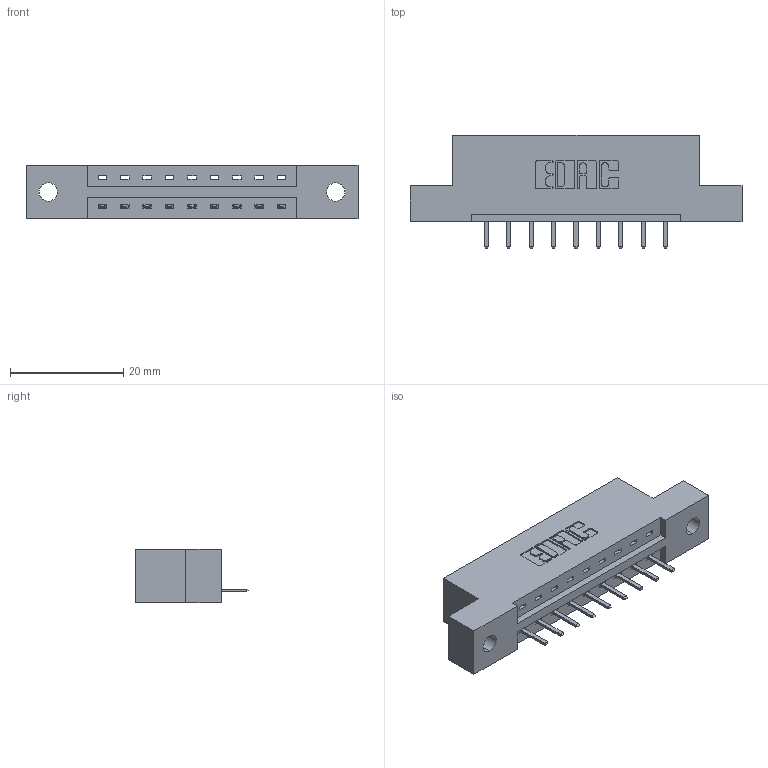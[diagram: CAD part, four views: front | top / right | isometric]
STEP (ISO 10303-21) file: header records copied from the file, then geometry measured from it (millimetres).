
FILE_DESCRIPTION (( 'STEP AP203' ), '1' );
FILE_NAME ('387-009-520-102.STEP', '2019-10-02T04:27:10', ( '' ), ( '' ), 'SwSTEP 2.0', 'SolidWorks 2016', '' );
FILE_SCHEMA (( 'CONFIG_CONTROL_DESIGN' ));
Length unit declared in the file: inch
Products named in the file (3): 337 Part_Flush Mounting Lugs - 0.128 Dia; 345-292-001_345-293-120; 387-009-520-102
Assembly tree (10 placements, depth 2):
  387-009-520-102
    337 Part_Flush Mounting Lugs - 0.128 Dia
    345-292-001_345-293-120  x9
Bounding box: 58.67 x 20.02 x 9.4 mm (x, y, z)
Volume: 5622.6 mm3; surface area: 5264 mm2
Topology: 10 solids, 10 shells, 708 faces, 2075 edges, 1358 vertices
Faces by surface type: plane 502, cylinder 206
Entity records: 11075 total; most frequent: CARTESIAN_POINT 1945, ORIENTED_EDGE 1878, DIRECTION 1693, EDGE_CURVE 939, LINE 807, VECTOR 807, VERTEX_POINT 622, AXIS2_PLACEMENT_3D 443
